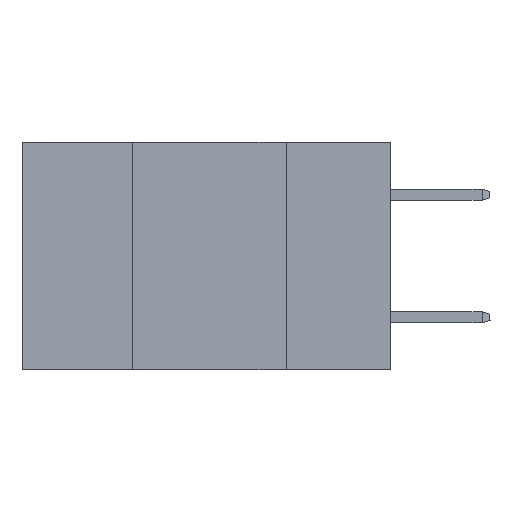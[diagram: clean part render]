
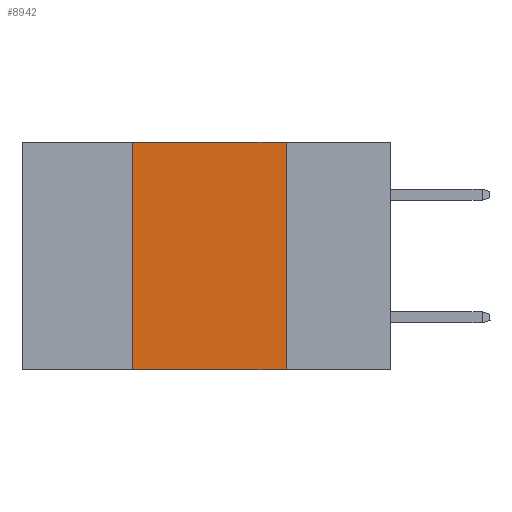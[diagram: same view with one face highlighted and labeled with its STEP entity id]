
A CAD part, left-side view. The second image highlights one B-rep face of the part: STEP entity #8942.
In plain terms, the highlighted planar face has unit normal (-1, 0, 0).
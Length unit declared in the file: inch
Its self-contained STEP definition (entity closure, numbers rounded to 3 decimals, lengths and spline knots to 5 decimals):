
#591 = CARTESIAN_POINT ( 'NONE',  ( 0., 0.17, 0. ) ) ;
#840 = CARTESIAN_POINT ( 'NONE',  ( 0., 0.6, 0. ) ) ;
#1485 = AXIS2_PLACEMENT_3D ( 'NONE', #840, #13027, #10612 ) ;
#2989 = EDGE_CURVE ( 'NONE', #7838, #13557, #4541, .T. ) ;
#3636 = EDGE_CURVE ( 'NONE', #8466, #13557, #8987, .T. ) ;
#4541 = LINE ( 'NONE', #9576, #15510 ) ;
#5100 = LINE ( 'NONE', #14674, #7074 ) ;
#5797 = EDGE_LOOP ( 'NONE', ( #8552, #6665, #9317, #12387 ) ) ;
#6226 = CARTESIAN_POINT ( 'NONE',  ( 0., 0.17, -0.37 ) ) ;
#6595 = LINE ( 'NONE', #13984, #15380 ) ;
#6665 = ORIENTED_EDGE ( 'NONE', *, *, #14926, .F. ) ;
#7074 = VECTOR ( 'NONE', #9811, 39.37008 ) ;
#7762 = VECTOR ( 'NONE', #10287, 39.37008 ) ;
#7838 = VERTEX_POINT ( 'NONE', #9002 ) ;
#8466 = VERTEX_POINT ( 'NONE', #591 ) ;
#8552 = ORIENTED_EDGE ( 'NONE', *, *, #3636, .F. ) ;
#8942 = ADVANCED_FACE ( 'NONE', ( #13350 ), #9463, .F. ) ;
#8987 = LINE ( 'NONE', #13932, #7762 ) ;
#9002 = CARTESIAN_POINT ( 'NONE',  ( 0., 0.42, -0.37 ) ) ;
#9317 = ORIENTED_EDGE ( 'NONE', *, *, #11022, .F. ) ;
#9463 = PLANE ( 'NONE',  #1485 ) ;
#9500 = DIRECTION ( 'NONE',  ( 0., -1., 0. ) ) ;
#9576 = CARTESIAN_POINT ( 'NONE',  ( 0., 0.6, -0.37 ) ) ;
#9811 = DIRECTION ( 'NONE',  ( 0., -1., 0. ) ) ;
#10287 = DIRECTION ( 'NONE',  ( 0., 0., -1. ) ) ;
#10612 = DIRECTION ( 'NONE',  ( 0., 0., -1. ) ) ;
#11022 = EDGE_CURVE ( 'NONE', #7838, #13745, #6595, .T. ) ;
#12387 = ORIENTED_EDGE ( 'NONE', *, *, #2989, .T. ) ;
#12563 = CARTESIAN_POINT ( 'NONE',  ( 0., 0.42, 0. ) ) ;
#12762 = DIRECTION ( 'NONE',  ( 0., 0., 1. ) ) ;
#13027 = DIRECTION ( 'NONE',  ( 1., 0., 0. ) ) ;
#13350 = FACE_OUTER_BOUND ( 'NONE', #5797, .T. ) ;
#13557 = VERTEX_POINT ( 'NONE', #6226 ) ;
#13745 = VERTEX_POINT ( 'NONE', #12563 ) ;
#13932 = CARTESIAN_POINT ( 'NONE',  ( 0., 0.17, 0. ) ) ;
#13984 = CARTESIAN_POINT ( 'NONE',  ( 0., 0.42, 0. ) ) ;
#14674 = CARTESIAN_POINT ( 'NONE',  ( 0., 0.6, 0. ) ) ;
#14926 = EDGE_CURVE ( 'NONE', #13745, #8466, #5100, .T. ) ;
#15380 = VECTOR ( 'NONE', #12762, 39.37008 ) ;
#15510 = VECTOR ( 'NONE', #9500, 39.37008 ) ;
